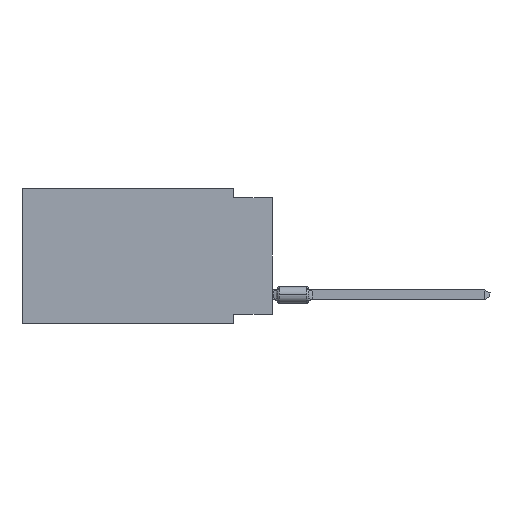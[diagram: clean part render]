
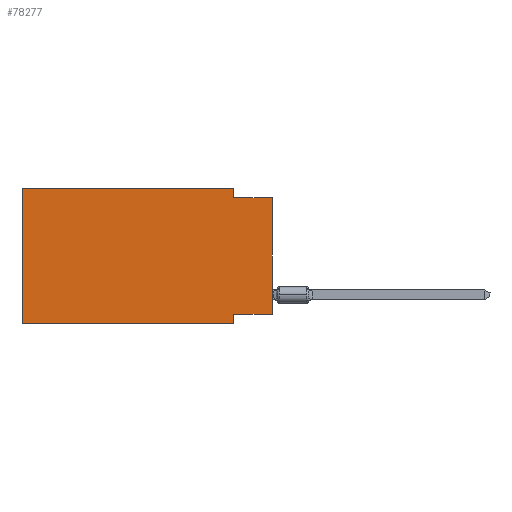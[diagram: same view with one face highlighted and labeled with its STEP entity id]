
A CAD part, left-side view. The second image highlights one B-rep face of the part: STEP entity #78277.
In plain terms, the highlighted planar face has unit normal (-1, 0, 0).
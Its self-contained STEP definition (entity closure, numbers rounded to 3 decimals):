
#144 = CARTESIAN_POINT ( 'NONE',  ( 0., 2.54, 0. ) ) ;
#8137 = VECTOR ( 'NONE', #34146, 1000. ) ;
#9190 = VECTOR ( 'NONE', #45301, 1000. ) ;
#11763 = DIRECTION ( 'NONE',  ( 1., 0., 0. ) ) ;
#11953 = EDGE_CURVE ( 'NONE', #22852, #56217, #49706, .T. ) ;
#13212 = EDGE_LOOP ( 'NONE', ( #83452, #32503, #44173, #81052, #69781, #73520, #19903, #67340 ) ) ;
#19629 = VECTOR ( 'NONE', #72496, 1000. ) ;
#19903 = ORIENTED_EDGE ( 'NONE', *, *, #61440, .F. ) ;
#19907 = EDGE_CURVE ( 'NONE', #43097, #22852, #43128, .T. ) ;
#21152 = VECTOR ( 'NONE', #42199, 1000. ) ;
#22852 = VERTEX_POINT ( 'NONE', #81245 ) ;
#27447 = DIRECTION ( 'NONE',  ( 0., -1., 0. ) ) ;
#28560 = VERTEX_POINT ( 'NONE', #77473 ) ;
#30747 = CARTESIAN_POINT ( 'NONE',  ( 0., 16.383, -8.89 ) ) ;
#32503 = ORIENTED_EDGE ( 'NONE', *, *, #67873, .F. ) ;
#34146 = DIRECTION ( 'NONE',  ( 0., 0., -1. ) ) ;
#34619 = CARTESIAN_POINT ( 'NONE',  ( 0., 16.383, 0. ) ) ;
#35498 = LINE ( 'NONE', #37706, #9190 ) ;
#35980 = AXIS2_PLACEMENT_3D ( 'NONE', #70003, #11763, #53481 ) ;
#36016 = CARTESIAN_POINT ( 'NONE',  ( 0., 2.54, 0. ) ) ;
#37387 = CARTESIAN_POINT ( 'NONE',  ( 0., 0., -8.255 ) ) ;
#37706 = CARTESIAN_POINT ( 'NONE',  ( 0., 0., 0. ) ) ;
#38333 = VECTOR ( 'NONE', #83447, 1000. ) ;
#41236 = CARTESIAN_POINT ( 'NONE',  ( 0., 2.54, -8.89 ) ) ;
#42199 = DIRECTION ( 'NONE',  ( 0., 0., 1. ) ) ;
#43097 = VERTEX_POINT ( 'NONE', #30747 ) ;
#43128 = LINE ( 'NONE', #34619, #21152 ) ;
#43627 = CARTESIAN_POINT ( 'NONE',  ( 0., 0., -0.635 ) ) ;
#44173 = ORIENTED_EDGE ( 'NONE', *, *, #48577, .F. ) ;
#45301 = DIRECTION ( 'NONE',  ( 0., 0., 1. ) ) ;
#48577 = EDGE_CURVE ( 'NONE', #56217, #28560, #58286, .T. ) ;
#49576 = EDGE_CURVE ( 'NONE', #61631, #59389, #35498, .T. ) ;
#49706 = LINE ( 'NONE', #55884, #86678 ) ;
#50231 = VERTEX_POINT ( 'NONE', #75459 ) ;
#53481 = DIRECTION ( 'NONE',  ( 0., 0., -1. ) ) ;
#54609 = CARTESIAN_POINT ( 'NONE',  ( 0., 0., -8.255 ) ) ;
#55884 = CARTESIAN_POINT ( 'NONE',  ( 0., 16.383, 0. ) ) ;
#56217 = VERTEX_POINT ( 'NONE', #144 ) ;
#58286 = LINE ( 'NONE', #36016, #67985 ) ;
#58750 = DIRECTION ( 'NONE',  ( 0., 0., -1. ) ) ;
#59389 = VERTEX_POINT ( 'NONE', #60849 ) ;
#60849 = CARTESIAN_POINT ( 'NONE',  ( 0., 0., -0.635 ) ) ;
#61440 = EDGE_CURVE ( 'NONE', #50231, #66534, #77224, .T. ) ;
#61631 = VERTEX_POINT ( 'NONE', #37387 ) ;
#63184 = LINE ( 'NONE', #43627, #19629 ) ;
#66022 = VECTOR ( 'NONE', #92196, 1000. ) ;
#66534 = VERTEX_POINT ( 'NONE', #69232 ) ;
#67340 = ORIENTED_EDGE ( 'NONE', *, *, #73315, .F. ) ;
#67873 = EDGE_CURVE ( 'NONE', #28560, #59389, #63184, .T. ) ;
#67985 = VECTOR ( 'NONE', #58750, 1000. ) ;
#69232 = CARTESIAN_POINT ( 'NONE',  ( 0., 2.54, -8.89 ) ) ;
#69781 = ORIENTED_EDGE ( 'NONE', *, *, #19907, .F. ) ;
#70003 = CARTESIAN_POINT ( 'NONE',  ( 0., 16.383, 0. ) ) ;
#70917 = CARTESIAN_POINT ( 'NONE',  ( 0., 16.383, -8.89 ) ) ;
#71838 = LINE ( 'NONE', #70917, #66022 ) ;
#72496 = DIRECTION ( 'NONE',  ( 0., -1., 0. ) ) ;
#73315 = EDGE_CURVE ( 'NONE', #61631, #50231, #89151, .T. ) ;
#73520 = ORIENTED_EDGE ( 'NONE', *, *, #77306, .T. ) ;
#75459 = CARTESIAN_POINT ( 'NONE',  ( 0., 2.54, -8.255 ) ) ;
#77224 = LINE ( 'NONE', #41236, #8137 ) ;
#77306 = EDGE_CURVE ( 'NONE', #43097, #66534, #71838, .T. ) ;
#77473 = CARTESIAN_POINT ( 'NONE',  ( 0., 2.54, -0.635 ) ) ;
#78277 = ADVANCED_FACE ( 'NONE', ( #88494 ), #84192, .F. ) ;
#81052 = ORIENTED_EDGE ( 'NONE', *, *, #11953, .F. ) ;
#81245 = CARTESIAN_POINT ( 'NONE',  ( 0., 16.383, 0. ) ) ;
#83447 = DIRECTION ( 'NONE',  ( 0., 1., 0. ) ) ;
#83452 = ORIENTED_EDGE ( 'NONE', *, *, #49576, .T. ) ;
#84192 = PLANE ( 'NONE',  #35980 ) ;
#86678 = VECTOR ( 'NONE', #27447, 1000. ) ;
#88494 = FACE_OUTER_BOUND ( 'NONE', #13212, .T. ) ;
#89151 = LINE ( 'NONE', #54609, #38333 ) ;
#92196 = DIRECTION ( 'NONE',  ( 0., -1., 0. ) ) ;
